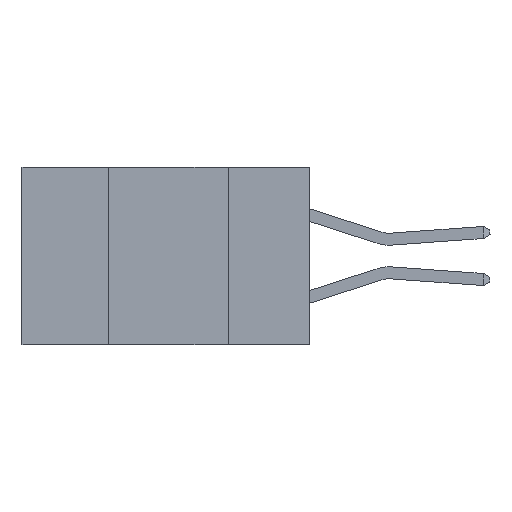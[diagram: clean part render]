
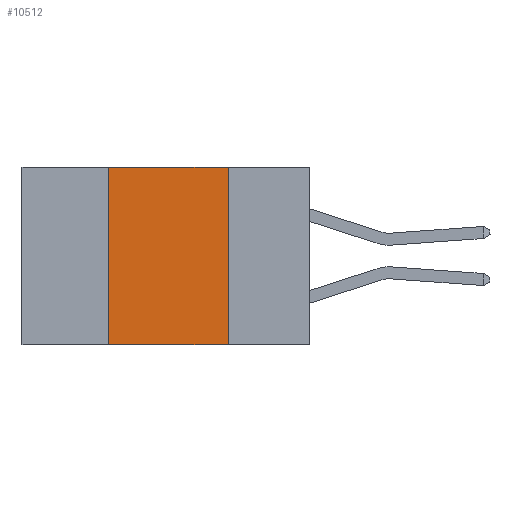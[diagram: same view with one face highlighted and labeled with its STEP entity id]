
A CAD part, left-side view. The second image highlights one B-rep face of the part: STEP entity #10512.
In plain terms, the highlighted planar face has unit normal (-1, 0, 0).
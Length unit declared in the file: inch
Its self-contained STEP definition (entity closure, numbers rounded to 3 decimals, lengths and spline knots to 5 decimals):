
#244 = VECTOR ( 'NONE', #9144, 39.37008 ) ;
#552 = PLANE ( 'NONE',  #729 ) ;
#729 = AXIS2_PLACEMENT_3D ( 'NONE', #10786, #9084, #2510 ) ;
#763 = CARTESIAN_POINT ( 'NONE',  ( 0., 0.6, 0. ) ) ;
#801 = DIRECTION ( 'NONE',  ( 0., -1., 0. ) ) ;
#1575 = LINE ( 'NONE', #4501, #244 ) ;
#1660 = VERTEX_POINT ( 'NONE', #10649 ) ;
#1805 = EDGE_CURVE ( 'NONE', #8140, #10537, #11200, .T. ) ;
#2023 = FACE_OUTER_BOUND ( 'NONE', #4043, .T. ) ;
#2092 = DIRECTION ( 'NONE',  ( 0., 0., -1. ) ) ;
#2510 = DIRECTION ( 'NONE',  ( 0., 0., -1. ) ) ;
#3462 = CARTESIAN_POINT ( 'NONE',  ( 0., 0.17, 0. ) ) ;
#4043 = EDGE_LOOP ( 'NONE', ( #10742, #4929, #9481, #11799 ) ) ;
#4069 = LINE ( 'NONE', #11327, #7863 ) ;
#4501 = CARTESIAN_POINT ( 'NONE',  ( 0., 0.6, -0.37 ) ) ;
#4929 = ORIENTED_EDGE ( 'NONE', *, *, #1805, .F. ) ;
#5194 = VECTOR ( 'NONE', #7829, 39.37008 ) ;
#5849 = CARTESIAN_POINT ( 'NONE',  ( 0., 0.42, 0. ) ) ;
#6169 = CARTESIAN_POINT ( 'NONE',  ( 0., 0.17, -0.37 ) ) ;
#6197 = EDGE_CURVE ( 'NONE', #1660, #8140, #9113, .T. ) ;
#7829 = DIRECTION ( 'NONE',  ( 0., 0., 1. ) ) ;
#7863 = VECTOR ( 'NONE', #2092, 39.37008 ) ;
#8140 = VERTEX_POINT ( 'NONE', #11465 ) ;
#9084 = DIRECTION ( 'NONE',  ( 1., 0., 0. ) ) ;
#9113 = LINE ( 'NONE', #5849, #5194 ) ;
#9144 = DIRECTION ( 'NONE',  ( 0., -1., 0. ) ) ;
#9481 = ORIENTED_EDGE ( 'NONE', *, *, #6197, .F. ) ;
#9482 = EDGE_CURVE ( 'NONE', #10537, #10569, #4069, .T. ) ;
#10194 = VECTOR ( 'NONE', #801, 39.37008 ) ;
#10512 = ADVANCED_FACE ( 'NONE', ( #2023 ), #552, .F. ) ;
#10537 = VERTEX_POINT ( 'NONE', #3462 ) ;
#10569 = VERTEX_POINT ( 'NONE', #6169 ) ;
#10649 = CARTESIAN_POINT ( 'NONE',  ( 0., 0.42, -0.37 ) ) ;
#10742 = ORIENTED_EDGE ( 'NONE', *, *, #9482, .F. ) ;
#10786 = CARTESIAN_POINT ( 'NONE',  ( 0., 0.6, 0. ) ) ;
#11200 = LINE ( 'NONE', #763, #10194 ) ;
#11327 = CARTESIAN_POINT ( 'NONE',  ( 0., 0.17, 0. ) ) ;
#11465 = CARTESIAN_POINT ( 'NONE',  ( 0., 0.42, 0. ) ) ;
#11799 = ORIENTED_EDGE ( 'NONE', *, *, #11861, .T. ) ;
#11861 = EDGE_CURVE ( 'NONE', #1660, #10569, #1575, .T. ) ;
